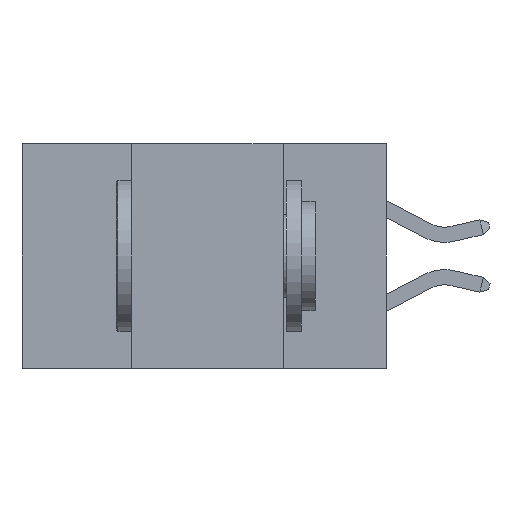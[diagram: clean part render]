
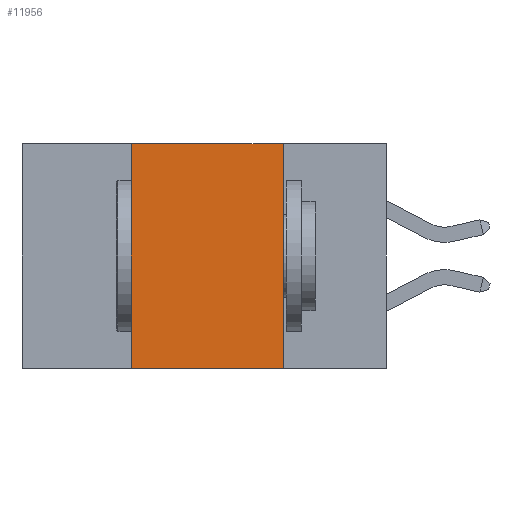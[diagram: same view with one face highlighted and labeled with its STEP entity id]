
A CAD part, left-side view. The second image highlights one B-rep face of the part: STEP entity #11956.
In plain terms, the highlighted planar face has unit normal (-1, 0, 0).
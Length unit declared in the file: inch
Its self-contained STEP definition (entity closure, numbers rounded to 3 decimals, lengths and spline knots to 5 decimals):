
#123 = VERTEX_POINT ( 'NONE', #5406 ) ;
#1406 = EDGE_CURVE ( 'NONE', #1764, #5014, #11517, .T. ) ;
#1442 = DIRECTION ( 'NONE',  ( 0., -1., 0. ) ) ;
#1541 = CARTESIAN_POINT ( 'NONE',  ( 0., 0.6, -0.37 ) ) ;
#1754 = CARTESIAN_POINT ( 'NONE',  ( 0., 0.6, 0. ) ) ;
#1764 = VERTEX_POINT ( 'NONE', #6587 ) ;
#2325 = VECTOR ( 'NONE', #2760, 39.37008 ) ;
#2731 = CARTESIAN_POINT ( 'NONE',  ( 0., 0.17, -0.37 ) ) ;
#2760 = DIRECTION ( 'NONE',  ( 0., 0., 1. ) ) ;
#2861 = DIRECTION ( 'NONE',  ( 0., 0., -1. ) ) ;
#3459 = VECTOR ( 'NONE', #4571, 39.37008 ) ;
#3497 = VECTOR ( 'NONE', #6586, 39.37008 ) ;
#4571 = DIRECTION ( 'NONE',  ( 0., -1., 0. ) ) ;
#4831 = LINE ( 'NONE', #6530, #2325 ) ;
#4886 = FACE_OUTER_BOUND ( 'NONE', #13559, .T. ) ;
#5014 = VERTEX_POINT ( 'NONE', #2731 ) ;
#5406 = CARTESIAN_POINT ( 'NONE',  ( 0., 0.42, 0. ) ) ;
#5700 = CARTESIAN_POINT ( 'NONE',  ( 0., 0.6, 0. ) ) ;
#5912 = EDGE_CURVE ( 'NONE', #123, #1764, #6213, .T. ) ;
#6080 = EDGE_CURVE ( 'NONE', #9486, #5014, #7343, .T. ) ;
#6213 = LINE ( 'NONE', #5700, #3459 ) ;
#6225 = ORIENTED_EDGE ( 'NONE', *, *, #6080, .T. ) ;
#6530 = CARTESIAN_POINT ( 'NONE',  ( 0., 0.42, -0.37 ) ) ;
#6550 = ORIENTED_EDGE ( 'NONE', *, *, #10308, .F. ) ;
#6586 = DIRECTION ( 'NONE',  ( 0., 0., -1. ) ) ;
#6587 = CARTESIAN_POINT ( 'NONE',  ( 0., 0.17, 0. ) ) ;
#6688 = VECTOR ( 'NONE', #1442, 39.37008 ) ;
#6772 = CARTESIAN_POINT ( 'NONE',  ( 0., 0.17, -0.37 ) ) ;
#7343 = LINE ( 'NONE', #1541, #6688 ) ;
#9180 = DIRECTION ( 'NONE',  ( 1., 0., 0. ) ) ;
#9393 = ORIENTED_EDGE ( 'NONE', *, *, #5912, .F. ) ;
#9486 = VERTEX_POINT ( 'NONE', #9488 ) ;
#9488 = CARTESIAN_POINT ( 'NONE',  ( 0., 0.42, -0.37 ) ) ;
#9509 = AXIS2_PLACEMENT_3D ( 'NONE', #1754, #9180, #2861 ) ;
#10308 = EDGE_CURVE ( 'NONE', #9486, #123, #4831, .T. ) ;
#11517 = LINE ( 'NONE', #6772, #3497 ) ;
#11956 = ADVANCED_FACE ( 'NONE', ( #4886 ), #13197, .F. ) ;
#12452 = ORIENTED_EDGE ( 'NONE', *, *, #1406, .F. ) ;
#13197 = PLANE ( 'NONE',  #9509 ) ;
#13559 = EDGE_LOOP ( 'NONE', ( #12452, #9393, #6550, #6225 ) ) ;
